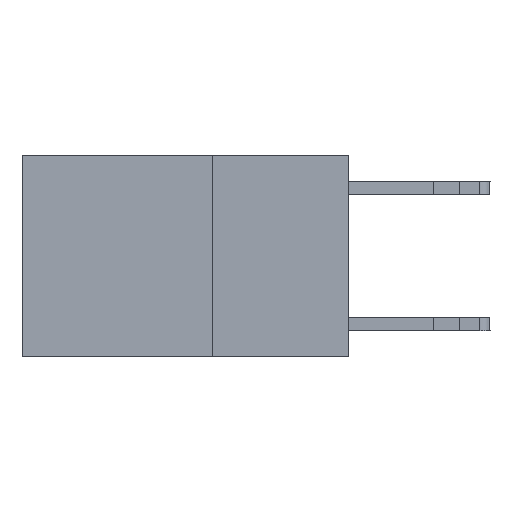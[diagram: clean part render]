
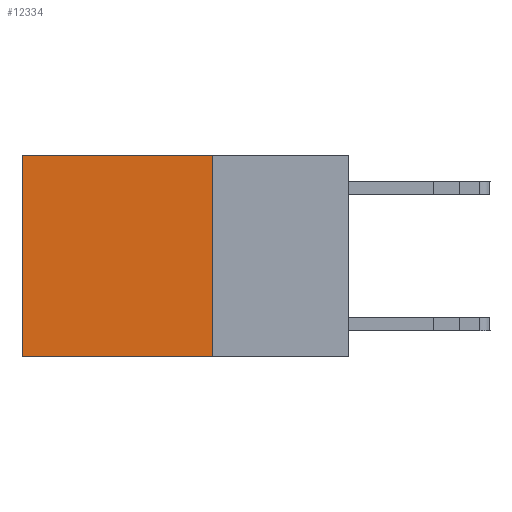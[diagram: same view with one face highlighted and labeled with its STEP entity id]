
A CAD part, left-side view. The second image highlights one B-rep face of the part: STEP entity #12334.
In plain terms, the highlighted planar face has unit normal (-1, 0, 0).
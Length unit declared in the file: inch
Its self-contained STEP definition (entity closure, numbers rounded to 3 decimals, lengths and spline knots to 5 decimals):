
#165 = EDGE_CURVE ( 'NONE', #26903, #11564, #17380, .T. ) ;
#529 = VERTEX_POINT ( 'NONE', #10179 ) ;
#685 = VERTEX_POINT ( 'NONE', #11985 ) ;
#1215 = PLANE ( 'NONE',  #16890 ) ;
#1443 = EDGE_CURVE ( 'NONE', #529, #685, #2495, .T. ) ;
#1992 = DIRECTION ( 'NONE',  ( 0., 0., -1. ) ) ;
#2351 = VECTOR ( 'NONE', #7443, 39.37008 ) ;
#2495 = LINE ( 'NONE', #11387, #9869 ) ;
#3474 = FACE_OUTER_BOUND ( 'NONE', #14748, .T. ) ;
#5319 = ORIENTED_EDGE ( 'NONE', *, *, #1443, .F. ) ;
#5982 = CARTESIAN_POINT ( 'NONE',  ( 0.2625, 0.25, 0. ) ) ;
#6429 = VECTOR ( 'NONE', #1992, 39.37008 ) ;
#6815 = DIRECTION ( 'NONE',  ( 0., 1., 0. ) ) ;
#7443 = DIRECTION ( 'NONE',  ( 0., 0., -1. ) ) ;
#8869 = CARTESIAN_POINT ( 'NONE',  ( 0.2625, 0.6, 0. ) ) ;
#9347 = ORIENTED_EDGE ( 'NONE', *, *, #9540, .F. ) ;
#9540 = EDGE_CURVE ( 'NONE', #26903, #529, #10177, .T. ) ;
#9869 = VECTOR ( 'NONE', #24056, 39.37008 ) ;
#10177 = LINE ( 'NONE', #18772, #6429 ) ;
#10179 = CARTESIAN_POINT ( 'NONE',  ( 0.2625, 0.25, -0.37 ) ) ;
#10380 = ORIENTED_EDGE ( 'NONE', *, *, #165, .T. ) ;
#11387 = CARTESIAN_POINT ( 'NONE',  ( 0.2625, 0.25, -0.37 ) ) ;
#11564 = VERTEX_POINT ( 'NONE', #8869 ) ;
#11985 = CARTESIAN_POINT ( 'NONE',  ( 0.2625, 0.6, -0.37 ) ) ;
#12249 = CARTESIAN_POINT ( 'NONE',  ( 0.2625, 0.6, 0. ) ) ;
#12334 = ADVANCED_FACE ( 'NONE', ( #3474 ), #1215, .F. ) ;
#12530 = ORIENTED_EDGE ( 'NONE', *, *, #19328, .T. ) ;
#14748 = EDGE_LOOP ( 'NONE', ( #12530, #5319, #9347, #10380 ) ) ;
#16890 = AXIS2_PLACEMENT_3D ( 'NONE', #5982, #27121, #23045 ) ;
#17380 = LINE ( 'NONE', #19364, #21592 ) ;
#18772 = CARTESIAN_POINT ( 'NONE',  ( 0.2625, 0.25, 0. ) ) ;
#19328 = EDGE_CURVE ( 'NONE', #11564, #685, #22810, .T. ) ;
#19364 = CARTESIAN_POINT ( 'NONE',  ( 0.2625, 0.25, 0. ) ) ;
#21592 = VECTOR ( 'NONE', #6815, 39.37008 ) ;
#22810 = LINE ( 'NONE', #12249, #2351 ) ;
#23045 = DIRECTION ( 'NONE',  ( 0., 0., -1. ) ) ;
#24056 = DIRECTION ( 'NONE',  ( 0., 1., 0. ) ) ;
#26420 = CARTESIAN_POINT ( 'NONE',  ( 0.2625, 0.25, 0. ) ) ;
#26903 = VERTEX_POINT ( 'NONE', #26420 ) ;
#27121 = DIRECTION ( 'NONE',  ( 1., 0., 0. ) ) ;
